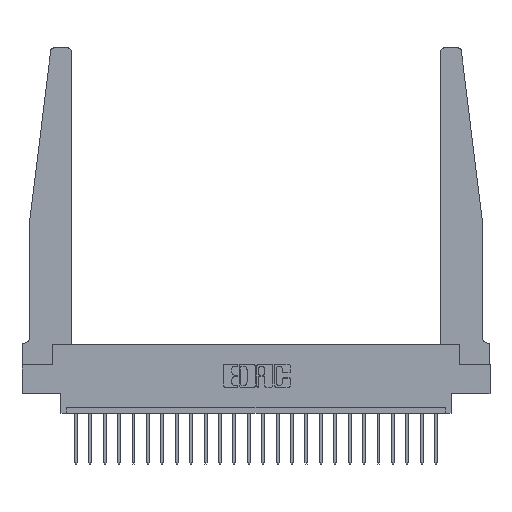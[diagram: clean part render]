
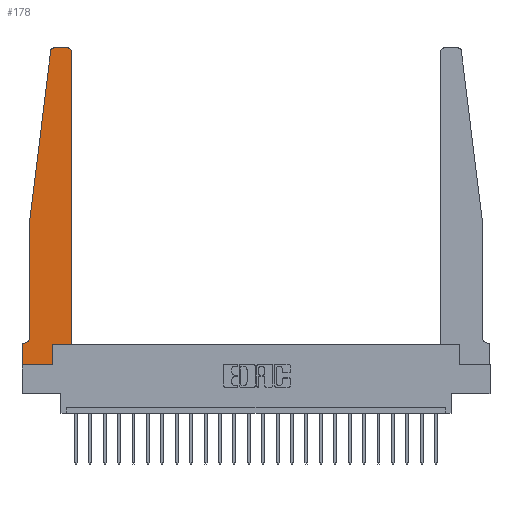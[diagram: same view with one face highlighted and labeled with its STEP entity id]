
A CAD part, top view. The second image highlights one B-rep face of the part: STEP entity #178.
In plain terms, the highlighted planar face has unit normal (0, 0, 1).
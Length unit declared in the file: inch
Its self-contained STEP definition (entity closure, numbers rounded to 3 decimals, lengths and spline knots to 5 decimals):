
#16 = EDGE_CURVE ( 'NONE', #11599, #10326, #17033, .T. ) ;
#178 = ADVANCED_FACE ( 'NONE', ( #17596 ), #1189, .T. ) ;
#198 = DIRECTION ( 'NONE',  ( 1., 0., 0. ) ) ;
#224 = ORIENTED_EDGE ( 'NONE', *, *, #10988, .T. ) ;
#249 = LINE ( 'NONE', #20137, #6948 ) ;
#537 = CARTESIAN_POINT ( 'NONE',  ( 0.27653, 2.75, 0.37 ) ) ;
#849 = EDGE_CURVE ( 'NONE', #8197, #21839, #22536, .T. ) ;
#871 = VECTOR ( 'NONE', #21919, 39.37008 ) ;
#961 = ORIENTED_EDGE ( 'NONE', *, *, #21727, .T. ) ;
#1189 = PLANE ( 'NONE',  #14744 ) ;
#1816 = CARTESIAN_POINT ( 'NONE',  ( 0., 0., 0.37 ) ) ;
#4030 = VERTEX_POINT ( 'NONE', #22201 ) ;
#4692 = ORIENTED_EDGE ( 'NONE', *, *, #14376, .T. ) ;
#4979 = EDGE_CURVE ( 'NONE', #17463, #17857, #5426, .T. ) ;
#5319 = EDGE_CURVE ( 'NONE', #17751, #11599, #19992, .T. ) ;
#5426 = LINE ( 'NONE', #1816, #871 ) ;
#5507 = VERTEX_POINT ( 'NONE', #18770 ) ;
#6082 = CIRCLE ( 'NONE', #19104, 0.05 ) ;
#6149 = CARTESIAN_POINT ( 'NONE',  ( 0.065, 1.25, 0.37 ) ) ;
#6609 = CARTESIAN_POINT ( 'NONE',  ( 0.2605, 0.18, 0.37 ) ) ;
#6948 = VECTOR ( 'NONE', #22038, 39.37008 ) ;
#7043 = EDGE_CURVE ( 'NONE', #5507, #22608, #18743, .T. ) ;
#7065 = ORIENTED_EDGE ( 'NONE', *, *, #16, .T. ) ;
#7365 = CARTESIAN_POINT ( 'NONE',  ( 0.24675, 2.72367, 0.37 ) ) ;
#7496 = DIRECTION ( 'NONE',  ( 0., 0., 1. ) ) ;
#7563 = VECTOR ( 'NONE', #16814, 39.37008 ) ;
#8170 = DIRECTION ( 'NONE',  ( 0., -1., 0. ) ) ;
#8197 = VERTEX_POINT ( 'NONE', #10189 ) ;
#8217 = VERTEX_POINT ( 'NONE', #18507 ) ;
#8862 = CARTESIAN_POINT ( 'NONE',  ( 0.015, 0.2375, 0.37 ) ) ;
#9133 = EDGE_CURVE ( 'NONE', #8217, #9400, #18620, .T. ) ;
#9262 = CIRCLE ( 'NONE', #18061, 0.03 ) ;
#9400 = VERTEX_POINT ( 'NONE', #22024 ) ;
#9635 = VECTOR ( 'NONE', #18205, 39.37008 ) ;
#9726 = ORIENTED_EDGE ( 'NONE', *, *, #5319, .T. ) ;
#10189 = CARTESIAN_POINT ( 'NONE',  ( 0.065, 1.25, 0.37 ) ) ;
#10326 = VERTEX_POINT ( 'NONE', #7365 ) ;
#10341 = LINE ( 'NONE', #17642, #15854 ) ;
#10412 = CARTESIAN_POINT ( 'NONE',  ( 0.2605, 0., 0.37 ) ) ;
#10413 = CARTESIAN_POINT ( 'NONE',  ( 0., 0.1875, 0.37 ) ) ;
#10439 = CARTESIAN_POINT ( 'NONE',  ( 0., 0., 0.37 ) ) ;
#10568 = DIRECTION ( 'NONE',  ( 0., 1., 0. ) ) ;
#10732 = CARTESIAN_POINT ( 'NONE',  ( 0., 0.1875, 0.37 ) ) ;
#10896 = CARTESIAN_POINT ( 'NONE',  ( 0.25, 2.75, 0.37 ) ) ;
#10988 = EDGE_CURVE ( 'NONE', #22608, #17463, #10341, .T. ) ;
#11487 = CARTESIAN_POINT ( 'NONE',  ( 0.27653, 2.72, 0.37 ) ) ;
#11599 = VERTEX_POINT ( 'NONE', #537 ) ;
#11886 = ORIENTED_EDGE ( 'NONE', *, *, #9133, .T. ) ;
#12268 = VECTOR ( 'NONE', #21852, 39.37008 ) ;
#12721 = DIRECTION ( 'NONE',  ( 1., 0., 0. ) ) ;
#13155 = ORIENTED_EDGE ( 'NONE', *, *, #849, .T. ) ;
#13175 = CARTESIAN_POINT ( 'NONE',  ( 0.065, 0.2375, 0.37 ) ) ;
#13242 = VECTOR ( 'NONE', #19180, 39.37008 ) ;
#13387 = DIRECTION ( 'NONE',  ( 1., 0., 0. ) ) ;
#13501 = DIRECTION ( 'NONE',  ( 0., 0., 1. ) ) ;
#13592 = AXIS2_PLACEMENT_3D ( 'NONE', #11487, #13501, #13387 ) ;
#14376 = EDGE_CURVE ( 'NONE', #4030, #8217, #21932, .T. ) ;
#14506 = CARTESIAN_POINT ( 'NONE',  ( 0.395, 2.72, 0.37 ) ) ;
#14744 = AXIS2_PLACEMENT_3D ( 'NONE', #10413, #7496, #198 ) ;
#14784 = VECTOR ( 'NONE', #18359, 39.37008 ) ;
#14821 = CARTESIAN_POINT ( 'NONE',  ( 0.395, 2.75, 0.37 ) ) ;
#15016 = CARTESIAN_POINT ( 'NONE',  ( 0.065, 0.1875, 0.37 ) ) ;
#15469 = CARTESIAN_POINT ( 'NONE',  ( 0.425, 0.18, 0.37 ) ) ;
#15811 = EDGE_CURVE ( 'NONE', #17857, #4030, #19562, .T. ) ;
#15854 = VECTOR ( 'NONE', #8170, 39.37008 ) ;
#16154 = DIRECTION ( 'NONE',  ( -1., 0., 0. ) ) ;
#16814 = DIRECTION ( 'NONE',  ( 0., -1., 0. ) ) ;
#17033 = CIRCLE ( 'NONE', #13592, 0.03 ) ;
#17224 = ORIENTED_EDGE ( 'NONE', *, *, #18964, .T. ) ;
#17463 = VERTEX_POINT ( 'NONE', #10439 ) ;
#17596 = FACE_OUTER_BOUND ( 'NONE', #23003, .T. ) ;
#17642 = CARTESIAN_POINT ( 'NONE',  ( 0., 0., 0.37 ) ) ;
#17751 = VERTEX_POINT ( 'NONE', #14821 ) ;
#17843 = ORIENTED_EDGE ( 'NONE', *, *, #7043, .T. ) ;
#17857 = VERTEX_POINT ( 'NONE', #10412 ) ;
#18020 = CARTESIAN_POINT ( 'NONE',  ( 0.425, 0.18, 0.37 ) ) ;
#18061 = AXIS2_PLACEMENT_3D ( 'NONE', #14506, #21813, #12721 ) ;
#18205 = DIRECTION ( 'NONE',  ( -1., 0., 0. ) ) ;
#18245 = ORIENTED_EDGE ( 'NONE', *, *, #4979, .T. ) ;
#18359 = DIRECTION ( 'NONE',  ( 1., 0., 0. ) ) ;
#18507 = CARTESIAN_POINT ( 'NONE',  ( 0.425, 0.18, 0.37 ) ) ;
#18620 = LINE ( 'NONE', #15469, #13242 ) ;
#18673 = VECTOR ( 'NONE', #10568, 39.37008 ) ;
#18743 = LINE ( 'NONE', #15016, #12268 ) ;
#18770 = CARTESIAN_POINT ( 'NONE',  ( 0.015, 0.1875, 0.37 ) ) ;
#18964 = EDGE_CURVE ( 'NONE', #21839, #5507, #6082, .T. ) ;
#19104 = AXIS2_PLACEMENT_3D ( 'NONE', #8862, #19975, #16154 ) ;
#19180 = DIRECTION ( 'NONE',  ( 0., 1., 0. ) ) ;
#19562 = LINE ( 'NONE', #6609, #18673 ) ;
#19975 = DIRECTION ( 'NONE',  ( 0., 0., -1. ) ) ;
#19992 = LINE ( 'NONE', #10896, #9635 ) ;
#20137 = CARTESIAN_POINT ( 'NONE',  ( 0.065, 1.25, 0.37 ) ) ;
#20444 = ORIENTED_EDGE ( 'NONE', *, *, #21900, .T. ) ;
#21727 = EDGE_CURVE ( 'NONE', #9400, #17751, #9262, .T. ) ;
#21813 = DIRECTION ( 'NONE',  ( 0., 0., 1. ) ) ;
#21839 = VERTEX_POINT ( 'NONE', #13175 ) ;
#21852 = DIRECTION ( 'NONE',  ( -1., 0., 0. ) ) ;
#21900 = EDGE_CURVE ( 'NONE', #10326, #8197, #249, .T. ) ;
#21919 = DIRECTION ( 'NONE',  ( 1., 0., 0. ) ) ;
#21932 = LINE ( 'NONE', #18020, #14784 ) ;
#22024 = CARTESIAN_POINT ( 'NONE',  ( 0.425, 2.72, 0.37 ) ) ;
#22038 = DIRECTION ( 'NONE',  ( -0.122, -0.992, 0. ) ) ;
#22046 = ORIENTED_EDGE ( 'NONE', *, *, #15811, .T. ) ;
#22201 = CARTESIAN_POINT ( 'NONE',  ( 0.2605, 0.18, 0.37 ) ) ;
#22536 = LINE ( 'NONE', #6149, #7563 ) ;
#22608 = VERTEX_POINT ( 'NONE', #10732 ) ;
#23003 = EDGE_LOOP ( 'NONE', ( #9726, #7065, #20444, #13155, #17224, #17843, #224, #18245, #22046, #4692, #11886, #961 ) ) ;
